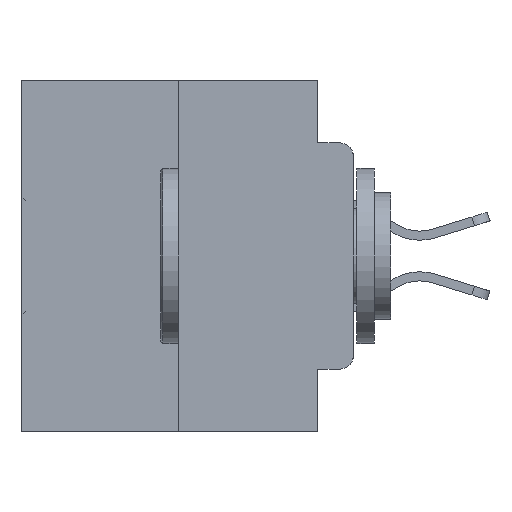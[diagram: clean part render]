
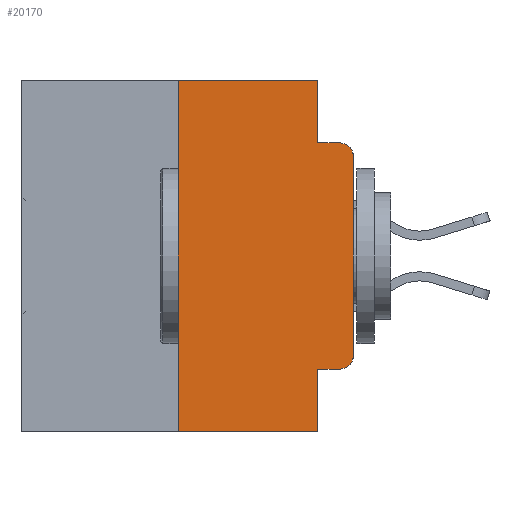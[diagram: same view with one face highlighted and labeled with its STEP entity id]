
A CAD part, left-side view. The second image highlights one B-rep face of the part: STEP entity #20170.
In plain terms, the highlighted planar face has unit normal (-1, 0, 0).
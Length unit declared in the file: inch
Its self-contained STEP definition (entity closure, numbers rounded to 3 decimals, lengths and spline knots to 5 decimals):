
#135 = CIRCLE ( 'NONE', #22629, 0.02 ) ;
#310 = CARTESIAN_POINT ( 'NONE',  ( 0., 0.051, 0. ) ) ;
#377 = VERTEX_POINT ( 'NONE', #13946 ) ;
#876 = CARTESIAN_POINT ( 'NONE',  ( 0., 0.051, -0.0885 ) ) ;
#998 = DIRECTION ( 'NONE',  ( 0., -1., 0. ) ) ;
#1269 = EDGE_LOOP ( 'NONE', ( #15091, #29091, #16642, #4050, #31397, #19002, #25602, #7271, #1280, #8832 ) ) ;
#1280 = ORIENTED_EDGE ( 'NONE', *, *, #22013, .T. ) ;
#1443 = EDGE_CURVE ( 'NONE', #4869, #5621, #6797, .T. ) ;
#1741 = LINE ( 'NONE', #13602, #27585 ) ;
#2151 = DIRECTION ( 'NONE',  ( -1., 0., 0. ) ) ;
#2398 = CARTESIAN_POINT ( 'NONE',  ( 0., 0.051, 0. ) ) ;
#2607 = VECTOR ( 'NONE', #7501, 39.37008 ) ;
#3139 = DIRECTION ( 'NONE',  ( -1., 0., 0. ) ) ;
#4050 = ORIENTED_EDGE ( 'NONE', *, *, #16833, .F. ) ;
#4869 = VERTEX_POINT ( 'NONE', #20396 ) ;
#5266 = CARTESIAN_POINT ( 'NONE',  ( 0., 0.051, 0. ) ) ;
#5621 = VERTEX_POINT ( 'NONE', #13651 ) ;
#5946 = CARTESIAN_POINT ( 'NONE',  ( 0., 0.25, -0.5 ) ) ;
#6781 = VECTOR ( 'NONE', #18490, 39.37008 ) ;
#6797 = LINE ( 'NONE', #9058, #14263 ) ;
#7271 = ORIENTED_EDGE ( 'NONE', *, *, #12450, .F. ) ;
#7501 = DIRECTION ( 'NONE',  ( 0., 0., -1. ) ) ;
#7599 = VERTEX_POINT ( 'NONE', #29036 ) ;
#8078 = DIRECTION ( 'NONE',  ( 0., -1., 0. ) ) ;
#8602 = VERTEX_POINT ( 'NONE', #5946 ) ;
#8832 = ORIENTED_EDGE ( 'NONE', *, *, #17033, .T. ) ;
#8885 = EDGE_CURVE ( 'NONE', #5621, #28741, #135, .T. ) ;
#8955 = DIRECTION ( 'NONE',  ( 0., 0., 1. ) ) ;
#9058 = CARTESIAN_POINT ( 'NONE',  ( 0., 0., 0. ) ) ;
#9088 = DIRECTION ( 'NONE',  ( 1., 0., 0. ) ) ;
#9653 = AXIS2_PLACEMENT_3D ( 'NONE', #18192, #3139, #20689 ) ;
#10273 = VECTOR ( 'NONE', #8078, 39.37008 ) ;
#10597 = VECTOR ( 'NONE', #20429, 39.37008 ) ;
#10758 = DIRECTION ( 'NONE',  ( 0., 0., 1. ) ) ;
#11056 = LINE ( 'NONE', #15530, #10273 ) ;
#11182 = EDGE_CURVE ( 'NONE', #21990, #28741, #13462, .T. ) ;
#11820 = EDGE_CURVE ( 'NONE', #8602, #14354, #29364, .T. ) ;
#12450 = EDGE_CURVE ( 'NONE', #377, #25594, #29706, .T. ) ;
#13462 = LINE ( 'NONE', #876, #6781 ) ;
#13602 = CARTESIAN_POINT ( 'NONE',  ( 0., 0.473, 0. ) ) ;
#13651 = CARTESIAN_POINT ( 'NONE',  ( 0., 0., -0.1085 ) ) ;
#13946 = CARTESIAN_POINT ( 'NONE',  ( 0., 0.051, -0.4115 ) ) ;
#14263 = VECTOR ( 'NONE', #8955, 39.37008 ) ;
#14354 = VERTEX_POINT ( 'NONE', #15646 ) ;
#15091 = ORIENTED_EDGE ( 'NONE', *, *, #1443, .T. ) ;
#15530 = CARTESIAN_POINT ( 'NONE',  ( 0., 0.473, -0.5 ) ) ;
#15646 = CARTESIAN_POINT ( 'NONE',  ( 0., 0.25, 0. ) ) ;
#16513 = PLANE ( 'NONE',  #21205 ) ;
#16642 = ORIENTED_EDGE ( 'NONE', *, *, #11182, .F. ) ;
#16833 = EDGE_CURVE ( 'NONE', #21336, #21990, #22589, .T. ) ;
#17033 = EDGE_CURVE ( 'NONE', #7599, #4869, #23742, .T. ) ;
#17217 = CARTESIAN_POINT ( 'NONE',  ( 0., 0.02, -0.1085 ) ) ;
#18192 = CARTESIAN_POINT ( 'NONE',  ( 0., 0.02, -0.3915 ) ) ;
#18490 = DIRECTION ( 'NONE',  ( 0., -1., 0. ) ) ;
#18584 = LINE ( 'NONE', #25237, #31768 ) ;
#19002 = ORIENTED_EDGE ( 'NONE', *, *, #11820, .F. ) ;
#19721 = CARTESIAN_POINT ( 'NONE',  ( 0., 0.051, -0.5 ) ) ;
#19724 = DIRECTION ( 'NONE',  ( 0., 0., -1. ) ) ;
#20170 = ADVANCED_FACE ( 'NONE', ( #20261 ), #16513, .F. ) ;
#20261 = FACE_OUTER_BOUND ( 'NONE', #1269, .T. ) ;
#20396 = CARTESIAN_POINT ( 'NONE',  ( 0., 0., -0.3915 ) ) ;
#20429 = DIRECTION ( 'NONE',  ( 0., 0., -1. ) ) ;
#20689 = DIRECTION ( 'NONE',  ( 0., 0., -1. ) ) ;
#21205 = AXIS2_PLACEMENT_3D ( 'NONE', #31380, #9088, #26510 ) ;
#21336 = VERTEX_POINT ( 'NONE', #5266 ) ;
#21825 = CARTESIAN_POINT ( 'NONE',  ( 0., 0.02, -0.0885 ) ) ;
#21990 = VERTEX_POINT ( 'NONE', #25127 ) ;
#22013 = EDGE_CURVE ( 'NONE', #377, #7599, #18584, .T. ) ;
#22589 = LINE ( 'NONE', #2398, #2607 ) ;
#22629 = AXIS2_PLACEMENT_3D ( 'NONE', #17217, #2151, #19724 ) ;
#23742 = CIRCLE ( 'NONE', #9653, 0.02 ) ;
#25127 = CARTESIAN_POINT ( 'NONE',  ( 0., 0.051, -0.0885 ) ) ;
#25237 = CARTESIAN_POINT ( 'NONE',  ( 0., 0.051, -0.4115 ) ) ;
#25594 = VERTEX_POINT ( 'NONE', #19721 ) ;
#25602 = ORIENTED_EDGE ( 'NONE', *, *, #28407, .T. ) ;
#25699 = CARTESIAN_POINT ( 'NONE',  ( 0., 0.25, 0. ) ) ;
#25970 = EDGE_CURVE ( 'NONE', #14354, #21336, #1741, .T. ) ;
#26510 = DIRECTION ( 'NONE',  ( 0., 0., -1. ) ) ;
#27585 = VECTOR ( 'NONE', #998, 39.37008 ) ;
#27727 = DIRECTION ( 'NONE',  ( 0., -1., 0. ) ) ;
#28407 = EDGE_CURVE ( 'NONE', #8602, #25594, #11056, .T. ) ;
#28569 = VECTOR ( 'NONE', #10758, 39.37008 ) ;
#28741 = VERTEX_POINT ( 'NONE', #21825 ) ;
#29036 = CARTESIAN_POINT ( 'NONE',  ( 0., 0.02, -0.4115 ) ) ;
#29091 = ORIENTED_EDGE ( 'NONE', *, *, #8885, .T. ) ;
#29364 = LINE ( 'NONE', #25699, #28569 ) ;
#29706 = LINE ( 'NONE', #310, #10597 ) ;
#31380 = CARTESIAN_POINT ( 'NONE',  ( 0., 0.473, 0. ) ) ;
#31397 = ORIENTED_EDGE ( 'NONE', *, *, #25970, .F. ) ;
#31768 = VECTOR ( 'NONE', #27727, 39.37008 ) ;
